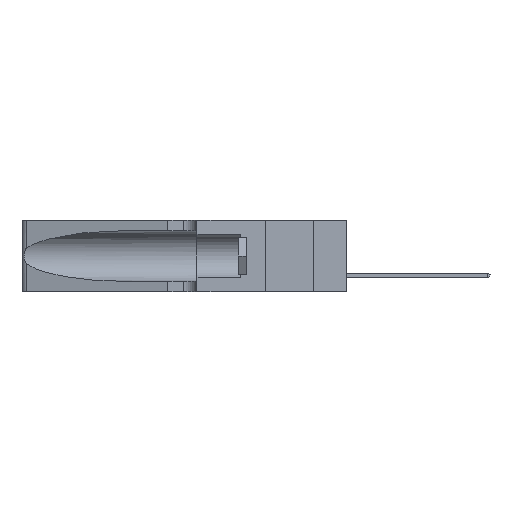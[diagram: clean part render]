
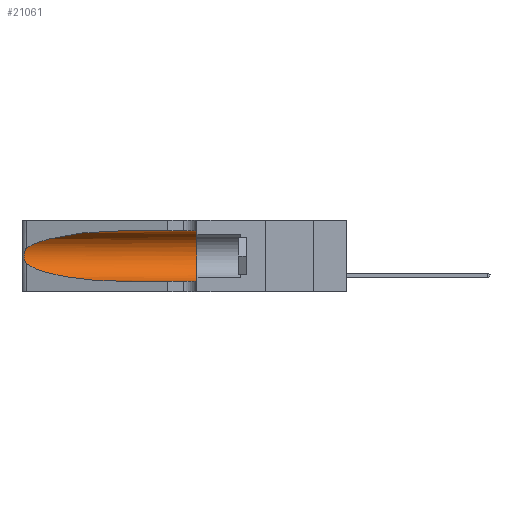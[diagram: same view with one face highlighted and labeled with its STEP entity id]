
A CAD part, left-side view. The second image highlights one B-rep face of the part: STEP entity #21061.
In plain terms, the highlighted cylindrical face has radius 3.308 mm (diameter 6.617 mm), a partial arc.
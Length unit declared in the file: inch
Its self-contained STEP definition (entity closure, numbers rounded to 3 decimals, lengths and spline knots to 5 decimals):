
#369 = FACE_OUTER_BOUND ( 'NONE', #25939, .T. ) ;
#527 = VECTOR ( 'NONE', #26326, 39.37008 ) ;
#811 = DIRECTION ( 'NONE',  ( 0., 1., 0. ) ) ;
#1649 = CIRCLE ( 'NONE', #28267, 0.13025 ) ;
#2206 = ORIENTED_EDGE ( 'NONE', *, *, #5770, .T. ) ;
#2295 = CARTESIAN_POINT ( 'NONE',  ( 0.1305, 0.72297, 0.05475 ) ) ;
#3120 = CARTESIAN_POINT ( 'NONE',  ( 0.25555, 1.22994, 0.2215 ) ) ;
#3534 = ORIENTED_EDGE ( 'NONE', *, *, #17977, .T. ) ;
#3786 = CARTESIAN_POINT ( 'NONE',  ( 0.25789, 1.23486, 0.15765 ) ) ;
#4344 = CARTESIAN_POINT ( 'NONE',  ( 0.25487, 1.22718, 0.14631 ) ) ;
#5587 = DIRECTION ( 'NONE',  ( 0., -1., 0. ) ) ;
#5703 =( BOUNDED_CURVE ( )  B_SPLINE_CURVE ( 3, ( #4344, #17832, #24520, #2295 ),
 .UNSPECIFIED., .F., .T. ) 
 B_SPLINE_CURVE_WITH_KNOTS ( ( 4, 4 ),
 ( 3.44316, 4.71239 ),
 .UNSPECIFIED. ) 
 CURVE ( )  GEOMETRIC_REPRESENTATION_ITEM ( )  RATIONAL_B_SPLINE_CURVE ( ( 1., 0.87, 0.87, 1. ) ) 
 REPRESENTATION_ITEM ( '' )  );
#5770 = EDGE_CURVE ( 'NONE', #12020, #20961, #5703, .T. ) ;
#5943 = CARTESIAN_POINT ( 'NONE',  ( 0.25854, 1.2359, 0.20912 ) ) ;
#6151 = CARTESIAN_POINT ( 'NONE',  ( 0.1305, 1.61858, 0.05475 ) ) ;
#6330 = EDGE_CURVE ( 'NONE', #20961, #18154, #11997, .T. ) ;
#8094 = CARTESIAN_POINT ( 'NONE',  ( 0.25639, 1.23184, 0.21858 ) ) ;
#8123 = DIRECTION ( 'NONE',  ( 0., -1., 0. ) ) ;
#8602 = VECTOR ( 'NONE', #5587, 39.37008 ) ;
#9332 = CARTESIAN_POINT ( 'NONE',  ( 0.25487, 1.22718, 0.22369 ) ) ;
#9381 = CYLINDRICAL_SURFACE ( 'NONE', #23075, 0.13025 ) ;
#9643 = ORIENTED_EDGE ( 'NONE', *, *, #10072, .F. ) ;
#10072 = EDGE_CURVE ( 'NONE', #18029, #15516, #11768, .T. ) ;
#10366 = CARTESIAN_POINT ( 'NONE',  ( 0.25856, 1.23593, 0.16098 ) ) ;
#10541 = ORIENTED_EDGE ( 'NONE', *, *, #10997, .F. ) ;
#10567 = CARTESIAN_POINT ( 'NONE',  ( 0.25639, 1.23186, 0.15144 ) ) ;
#10788 = CARTESIAN_POINT ( 'NONE',  ( 0.1305, 0.35, 0.31525 ) ) ;
#10997 = EDGE_CURVE ( 'NONE', #15516, #18154, #1649, .T. ) ;
#11768 = LINE ( 'NONE', #23266, #8602 ) ;
#11838 = CARTESIAN_POINT ( 'NONE',  ( 0.25487, 1.22718, 0.14631 ) ) ;
#11997 = LINE ( 'NONE', #6151, #527 ) ;
#12020 = VERTEX_POINT ( 'NONE', #11838 ) ;
#12718 = VERTEX_POINT ( 'NONE', #9332 ) ;
#13441 =( BOUNDED_CURVE ( )  B_SPLINE_CURVE ( 3, ( #18392, #15946, #26914, #20308 ),
 .UNSPECIFIED., .F., .F. ) 
 B_SPLINE_CURVE_WITH_KNOTS ( ( 4, 4 ),
 ( 1.5708, 2.84003 ),
 .UNSPECIFIED. ) 
 CURVE ( )  GEOMETRIC_REPRESENTATION_ITEM ( )  RATIONAL_B_SPLINE_CURVE ( ( 1., 0.87, 0.87, 1. ) ) 
 REPRESENTATION_ITEM ( '' )  );
#14512 = CARTESIAN_POINT ( 'NONE',  ( 0.1305, 1.61858, 0.185 ) ) ;
#15516 = VERTEX_POINT ( 'NONE', #10788 ) ;
#15946 = CARTESIAN_POINT ( 'NONE',  ( 0.18966, 0.96281, 0.31525 ) ) ;
#16388 = CARTESIAN_POINT ( 'NONE',  ( 0.1305, 0.72297, 0.31525 ) ) ;
#16857 = DIRECTION ( 'NONE',  ( 0., 0., -1. ) ) ;
#17832 = CARTESIAN_POINT ( 'NONE',  ( 0.2373, 1.15595, 0.08982 ) ) ;
#17977 = EDGE_CURVE ( 'NONE', #18029, #12718, #13441, .T. ) ;
#18029 = VERTEX_POINT ( 'NONE', #16388 ) ;
#18053 = ORIENTED_EDGE ( 'NONE', *, *, #20730, .T. ) ;
#18154 = VERTEX_POINT ( 'NONE', #19760 ) ;
#18392 = CARTESIAN_POINT ( 'NONE',  ( 0.1305, 0.72297, 0.31525 ) ) ;
#18743 = ORIENTED_EDGE ( 'NONE', *, *, #6330, .T. ) ;
#19760 = CARTESIAN_POINT ( 'NONE',  ( 0.1305, 0.35, 0.05475 ) ) ;
#20308 = CARTESIAN_POINT ( 'NONE',  ( 0.25487, 1.22718, 0.22369 ) ) ;
#20730 = EDGE_CURVE ( 'NONE', #12718, #12020, #25550, .T. ) ;
#20961 = VERTEX_POINT ( 'NONE', #27011 ) ;
#21061 = ADVANCED_FACE ( 'NONE', ( #369 ), #9381, .F. ) ;
#21352 = CARTESIAN_POINT ( 'NONE',  ( 0.26017, 1.23833, 0.17102 ) ) ;
#21501 = DIRECTION ( 'NONE',  ( 0., 0., 1. ) ) ;
#21542 = CARTESIAN_POINT ( 'NONE',  ( 0.26075, 1.23896, 0.19203 ) ) ;
#23075 = AXIS2_PLACEMENT_3D ( 'NONE', #14512, #8123, #16857 ) ;
#23266 = CARTESIAN_POINT ( 'NONE',  ( 0.1305, 1.61858, 0.31525 ) ) ;
#23381 = CARTESIAN_POINT ( 'NONE',  ( 0.1305, 0.35, 0.185 ) ) ;
#23609 = CARTESIAN_POINT ( 'NONE',  ( 0.25487, 1.22718, 0.14631 ) ) ;
#24520 = CARTESIAN_POINT ( 'NONE',  ( 0.18966, 0.96281, 0.05475 ) ) ;
#25550 = B_SPLINE_CURVE_WITH_KNOTS ( 'NONE', 3,
 ( #27928, #3120, #8094, #26213, #5943, #25837, #21542, #28208, #21352, #10366, #3786, #10567, #26116, #23609 ),
 .UNSPECIFIED., .F., .F.,
 ( 4, 2, 2, 2, 2, 2, 4 ),
 ( 0., 0.00027, 0.00053, 0.00107, 0.0016, 0.00187, 0.00214 ),
 .UNSPECIFIED. ) ;
#25837 = CARTESIAN_POINT ( 'NONE',  ( 0.26018, 1.23835, 0.19895 ) ) ;
#25939 = EDGE_LOOP ( 'NONE', ( #3534, #18053, #2206, #18743, #10541, #9643 ) ) ;
#26116 = CARTESIAN_POINT ( 'NONE',  ( 0.25555, 1.22993, 0.14849 ) ) ;
#26213 = CARTESIAN_POINT ( 'NONE',  ( 0.25787, 1.23484, 0.2124 ) ) ;
#26326 = DIRECTION ( 'NONE',  ( 0., -1., 0. ) ) ;
#26914 = CARTESIAN_POINT ( 'NONE',  ( 0.2373, 1.15595, 0.28018 ) ) ;
#27011 = CARTESIAN_POINT ( 'NONE',  ( 0.1305, 0.72297, 0.05475 ) ) ;
#27928 = CARTESIAN_POINT ( 'NONE',  ( 0.25487, 1.22718, 0.22369 ) ) ;
#28208 = CARTESIAN_POINT ( 'NONE',  ( 0.26075, 1.23896, 0.178 ) ) ;
#28267 = AXIS2_PLACEMENT_3D ( 'NONE', #23381, #811, #21501 ) ;
